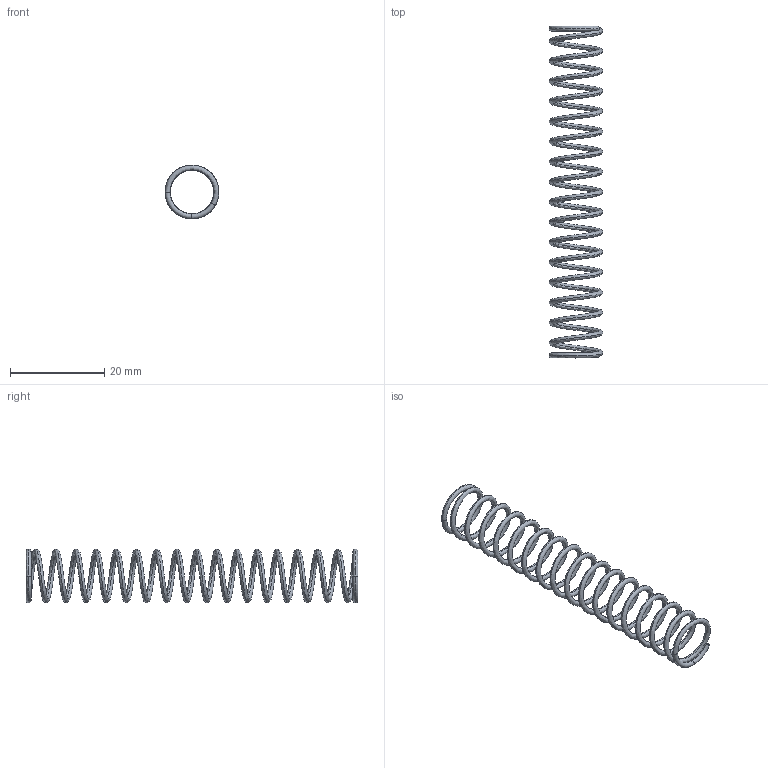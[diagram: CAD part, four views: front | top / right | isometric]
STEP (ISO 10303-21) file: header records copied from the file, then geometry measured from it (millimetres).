
FILE_DESCRIPTION (( 'STEP AP214' ), '1' );
FILE_NAME ('Recoil Spring.step', '2014-07-30T19:46:41', ( 'WarFairy' ), ( '' ), 'SwSTEP 2.0', 'SolidWorks 2013', '' );
FILE_SCHEMA (( 'AUTOMOTIVE_DESIGN' ));
Length unit declared in the file: millimetre
Products named in the file (1): Recoil Spring
Bounding box: 11.44 x 70.48 x 11.44 mm (x, y, z)
Volume: 518.8 mm3; surface area: 1952.4 mm2
Topology: 1 solids, 1 shells, 10 faces, 24 edges, 14 vertices
Faces by surface type: torus 4, bspline 4, plane 2
Entity records: 6287 total; most frequent: CARTESIAN_POINT 6051, ORIENTED_EDGE 48, DIRECTION 32, EDGE_CURVE 24, AXIS2_PLACEMENT_3D 16, VERTEX_POINT 14, B_SPLINE_CURVE_WITH_KNOTS 13, EDGE_LOOP 12
